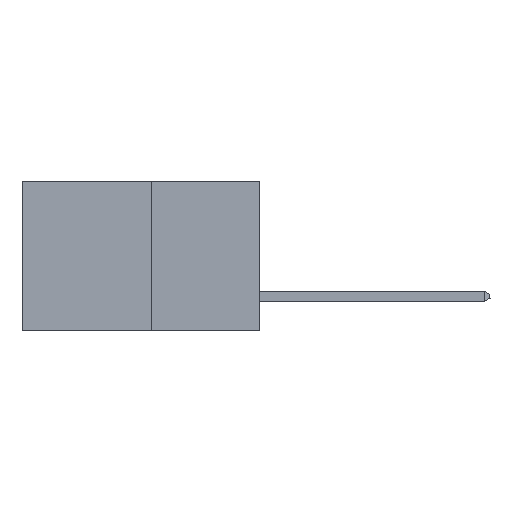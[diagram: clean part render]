
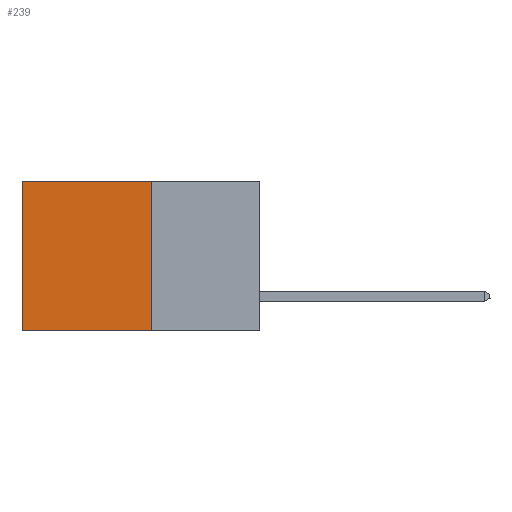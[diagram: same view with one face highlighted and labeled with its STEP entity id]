
A CAD part, left-side view. The second image highlights one B-rep face of the part: STEP entity #239.
In plain terms, the highlighted planar face has unit normal (-1, 0, 0).
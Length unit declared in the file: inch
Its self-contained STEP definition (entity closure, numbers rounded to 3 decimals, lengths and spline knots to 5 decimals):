
#239 = ADVANCED_FACE ( 'NONE', ( #14694 ), #8876, .F. ) ;
#1421 = VERTEX_POINT ( 'NONE', #5016 ) ;
#2502 = DIRECTION ( 'NONE',  ( 0., 0., -1. ) ) ;
#2541 = LINE ( 'NONE', #15260, #15364 ) ;
#2576 = CARTESIAN_POINT ( 'NONE',  ( 0.277, 0.59, -0.37 ) ) ;
#3524 = LINE ( 'NONE', #2576, #6515 ) ;
#4867 = CARTESIAN_POINT ( 'NONE',  ( 0.277, 0.27, -0.37 ) ) ;
#4911 = VECTOR ( 'NONE', #12777, 39.37008 ) ;
#5012 = ORIENTED_EDGE ( 'NONE', *, *, #10230, .T. ) ;
#5016 = CARTESIAN_POINT ( 'NONE',  ( 0.277, 0.59, 0. ) ) ;
#5309 = LINE ( 'NONE', #11354, #4911 ) ;
#5398 = VERTEX_POINT ( 'NONE', #10827 ) ;
#5473 = CARTESIAN_POINT ( 'NONE',  ( 0.277, 0.59, -0.37 ) ) ;
#5613 = ORIENTED_EDGE ( 'NONE', *, *, #5915, .F. ) ;
#5915 = EDGE_CURVE ( 'NONE', #5398, #8192, #5309, .T. ) ;
#6229 = VERTEX_POINT ( 'NONE', #5473 ) ;
#6515 = VECTOR ( 'NONE', #2502, 39.37008 ) ;
#6684 = DIRECTION ( 'NONE',  ( 0., 1., 0. ) ) ;
#7500 = EDGE_CURVE ( 'NONE', #5398, #1421, #11306, .T. ) ;
#7713 = DIRECTION ( 'NONE',  ( 0., 1., 0. ) ) ;
#7823 = CARTESIAN_POINT ( 'NONE',  ( 0.277, 0.27, 0. ) ) ;
#8052 = VECTOR ( 'NONE', #7713, 39.37008 ) ;
#8192 = VERTEX_POINT ( 'NONE', #4867 ) ;
#8853 = CARTESIAN_POINT ( 'NONE',  ( 0.277, 0.27, -0.37 ) ) ;
#8876 = PLANE ( 'NONE',  #11592 ) ;
#9492 = DIRECTION ( 'NONE',  ( 0., 0., -1. ) ) ;
#9509 = DIRECTION ( 'NONE',  ( 1., 0., 0. ) ) ;
#10230 = EDGE_CURVE ( 'NONE', #1421, #6229, #3524, .T. ) ;
#10827 = CARTESIAN_POINT ( 'NONE',  ( 0.277, 0.27, 0. ) ) ;
#11306 = LINE ( 'NONE', #7823, #8052 ) ;
#11354 = CARTESIAN_POINT ( 'NONE',  ( 0.277, 0.27, -0.37 ) ) ;
#11592 = AXIS2_PLACEMENT_3D ( 'NONE', #8853, #9509, #9492 ) ;
#12777 = DIRECTION ( 'NONE',  ( 0., 0., -1. ) ) ;
#13205 = EDGE_LOOP ( 'NONE', ( #5012, #13763, #5613, #13946 ) ) ;
#13763 = ORIENTED_EDGE ( 'NONE', *, *, #15185, .F. ) ;
#13946 = ORIENTED_EDGE ( 'NONE', *, *, #7500, .T. ) ;
#14694 = FACE_OUTER_BOUND ( 'NONE', #13205, .T. ) ;
#15185 = EDGE_CURVE ( 'NONE', #8192, #6229, #2541, .T. ) ;
#15260 = CARTESIAN_POINT ( 'NONE',  ( 0.277, 0.27, -0.37 ) ) ;
#15364 = VECTOR ( 'NONE', #6684, 39.37008 ) ;
